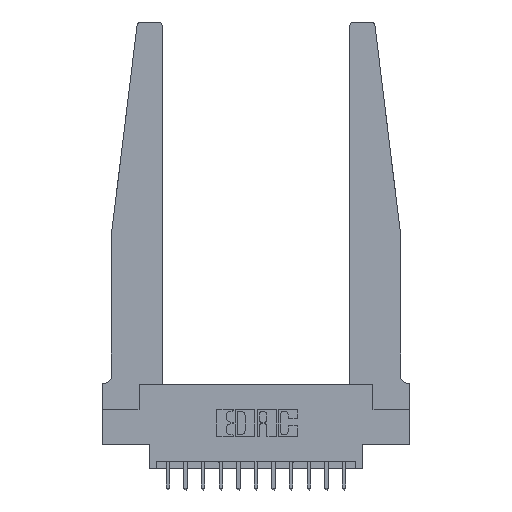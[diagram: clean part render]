
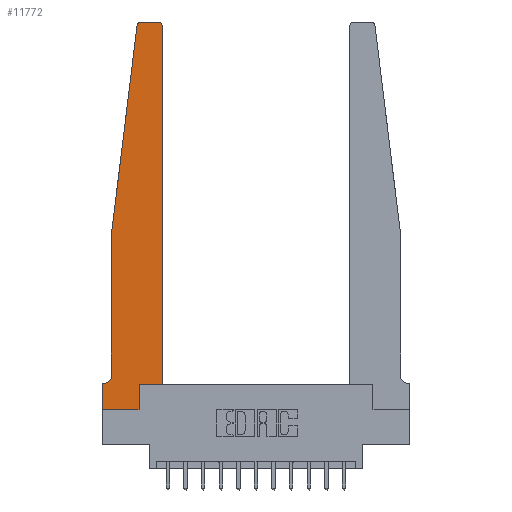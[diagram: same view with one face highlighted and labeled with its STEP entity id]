
A CAD part, top view. The second image highlights one B-rep face of the part: STEP entity #11772.
In plain terms, the highlighted planar face has unit normal (0, 0, 1).
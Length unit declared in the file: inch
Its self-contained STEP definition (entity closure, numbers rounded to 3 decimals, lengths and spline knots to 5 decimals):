
#385 = CARTESIAN_POINT ( 'NONE',  ( 0., 0., 0.37 ) ) ;
#514 = VERTEX_POINT ( 'NONE', #5692 ) ;
#535 = VERTEX_POINT ( 'NONE', #10889 ) ;
#647 = DIRECTION ( 'NONE',  ( 0., 0., -1. ) ) ;
#896 = DIRECTION ( 'NONE',  ( 0., 1., 0. ) ) ;
#1095 = LINE ( 'NONE', #7437, #6168 ) ;
#1302 = EDGE_CURVE ( 'NONE', #15750, #10964, #5642, .T. ) ;
#1675 = VECTOR ( 'NONE', #5531, 39.37008 ) ;
#1702 = VERTEX_POINT ( 'NONE', #1838 ) ;
#1838 = CARTESIAN_POINT ( 'NONE',  ( 0.2605, 0., 0.37 ) ) ;
#1905 = AXIS2_PLACEMENT_3D ( 'NONE', #12193, #647, #10921 ) ;
#1984 = CARTESIAN_POINT ( 'NONE',  ( 0.25, 2.75, 0.37 ) ) ;
#2105 = CARTESIAN_POINT ( 'NONE',  ( 0.2605, 0.18, 0.37 ) ) ;
#2109 = EDGE_CURVE ( 'NONE', #9796, #15750, #9863, .T. ) ;
#2188 = LINE ( 'NONE', #2105, #16376 ) ;
#2191 = VERTEX_POINT ( 'NONE', #4500 ) ;
#2265 = CARTESIAN_POINT ( 'NONE',  ( 0.065, 1.25, 0.37 ) ) ;
#2681 = VERTEX_POINT ( 'NONE', #16068 ) ;
#2759 = CARTESIAN_POINT ( 'NONE',  ( 0., 0., 0.37 ) ) ;
#2778 = VERTEX_POINT ( 'NONE', #15477 ) ;
#2953 = ORIENTED_EDGE ( 'NONE', *, *, #4439, .T. ) ;
#2957 = DIRECTION ( 'NONE',  ( 1., 0., 0. ) ) ;
#3005 = DIRECTION ( 'NONE',  ( -1., 0., 0. ) ) ;
#3137 = AXIS2_PLACEMENT_3D ( 'NONE', #9497, #13600, #11223 ) ;
#3328 = CARTESIAN_POINT ( 'NONE',  ( 0., 0., 0.37 ) ) ;
#3428 = ORIENTED_EDGE ( 'NONE', *, *, #8818, .T. ) ;
#3471 = ORIENTED_EDGE ( 'NONE', *, *, #4637, .T. ) ;
#4064 = EDGE_CURVE ( 'NONE', #535, #14645, #5435, .T. ) ;
#4354 = DIRECTION ( 'NONE',  ( -0.122, -0.992, 0. ) ) ;
#4439 = EDGE_CURVE ( 'NONE', #2778, #2681, #5940, .T. ) ;
#4500 = CARTESIAN_POINT ( 'NONE',  ( 0.2605, 0.18, 0.37 ) ) ;
#4637 = EDGE_CURVE ( 'NONE', #13039, #1702, #6805, .T. ) ;
#5165 = VECTOR ( 'NONE', #10981, 39.37008 ) ;
#5435 = CIRCLE ( 'NONE', #11888, 0.03 ) ;
#5531 = DIRECTION ( 'NONE',  ( 0., -1., 0. ) ) ;
#5535 = ORIENTED_EDGE ( 'NONE', *, *, #8652, .T. ) ;
#5642 = LINE ( 'NONE', #8272, #13247 ) ;
#5692 = CARTESIAN_POINT ( 'NONE',  ( 0.425, 0.18, 0.37 ) ) ;
#5865 = EDGE_CURVE ( 'NONE', #14645, #9796, #16175, .T. ) ;
#5940 = CIRCLE ( 'NONE', #1905, 0.05 ) ;
#6006 = VECTOR ( 'NONE', #13060, 39.37008 ) ;
#6052 = CARTESIAN_POINT ( 'NONE',  ( 0.24675, 2.72367, 0.37 ) ) ;
#6168 = VECTOR ( 'NONE', #16646, 39.37008 ) ;
#6522 = EDGE_CURVE ( 'NONE', #514, #535, #15718, .T. ) ;
#6621 = LINE ( 'NONE', #12861, #8922 ) ;
#6805 = LINE ( 'NONE', #2759, #9969 ) ;
#7226 = LINE ( 'NONE', #385, #1675 ) ;
#7437 = CARTESIAN_POINT ( 'NONE',  ( 0.425, 0.18, 0.37 ) ) ;
#7659 = CARTESIAN_POINT ( 'NONE',  ( 0.395, 2.75, 0.37 ) ) ;
#8180 = ORIENTED_EDGE ( 'NONE', *, *, #5865, .T. ) ;
#8272 = CARTESIAN_POINT ( 'NONE',  ( 0.065, 1.25, 0.37 ) ) ;
#8652 = EDGE_CURVE ( 'NONE', #10964, #2778, #6621, .T. ) ;
#8818 = EDGE_CURVE ( 'NONE', #9942, #13039, #7226, .T. ) ;
#8922 = VECTOR ( 'NONE', #11744, 39.37008 ) ;
#8942 = DIRECTION ( 'NONE',  ( 0., 0., 1. ) ) ;
#9103 = CARTESIAN_POINT ( 'NONE',  ( 0.395, 2.72, 0.37 ) ) ;
#9215 = ORIENTED_EDGE ( 'NONE', *, *, #1302, .T. ) ;
#9420 = LINE ( 'NONE', #14557, #12294 ) ;
#9497 = CARTESIAN_POINT ( 'NONE',  ( 0.27653, 2.72, 0.37 ) ) ;
#9796 = VERTEX_POINT ( 'NONE', #10140 ) ;
#9863 = CIRCLE ( 'NONE', #3137, 0.03 ) ;
#9942 = VERTEX_POINT ( 'NONE', #10730 ) ;
#9969 = VECTOR ( 'NONE', #14473, 39.37008 ) ;
#10069 = EDGE_LOOP ( 'NONE', ( #8180, #12235, #9215, #5535, #2953, #11363, #3428, #3471, #11829, #13147, #10459, #15110 ) ) ;
#10140 = CARTESIAN_POINT ( 'NONE',  ( 0.27653, 2.75, 0.37 ) ) ;
#10459 = ORIENTED_EDGE ( 'NONE', *, *, #6522, .T. ) ;
#10730 = CARTESIAN_POINT ( 'NONE',  ( 0., 0.1875, 0.37 ) ) ;
#10774 = EDGE_CURVE ( 'NONE', #1702, #2191, #2188, .T. ) ;
#10889 = CARTESIAN_POINT ( 'NONE',  ( 0.425, 2.72, 0.37 ) ) ;
#10921 = DIRECTION ( 'NONE',  ( -1., 0., 0. ) ) ;
#10964 = VERTEX_POINT ( 'NONE', #2265 ) ;
#10981 = DIRECTION ( 'NONE',  ( -1., 0., 0. ) ) ;
#11223 = DIRECTION ( 'NONE',  ( 1., 0., 0. ) ) ;
#11363 = ORIENTED_EDGE ( 'NONE', *, *, #13009, .T. ) ;
#11744 = DIRECTION ( 'NONE',  ( 0., -1., 0. ) ) ;
#11772 = ADVANCED_FACE ( 'NONE', ( #14340 ), #15967, .T. ) ;
#11829 = ORIENTED_EDGE ( 'NONE', *, *, #10774, .T. ) ;
#11873 = CARTESIAN_POINT ( 'NONE',  ( 0.425, 0.18, 0.37 ) ) ;
#11888 = AXIS2_PLACEMENT_3D ( 'NONE', #9103, #8942, #16634 ) ;
#12193 = CARTESIAN_POINT ( 'NONE',  ( 0.015, 0.2375, 0.37 ) ) ;
#12235 = ORIENTED_EDGE ( 'NONE', *, *, #2109, .T. ) ;
#12294 = VECTOR ( 'NONE', #3005, 39.37008 ) ;
#12861 = CARTESIAN_POINT ( 'NONE',  ( 0.065, 1.25, 0.37 ) ) ;
#13009 = EDGE_CURVE ( 'NONE', #2681, #9942, #9420, .T. ) ;
#13039 = VERTEX_POINT ( 'NONE', #3328 ) ;
#13060 = DIRECTION ( 'NONE',  ( 0., 1., 0. ) ) ;
#13062 = CARTESIAN_POINT ( 'NONE',  ( 0., 0.1875, 0.37 ) ) ;
#13147 = ORIENTED_EDGE ( 'NONE', *, *, #15438, .T. ) ;
#13247 = VECTOR ( 'NONE', #4354, 39.37008 ) ;
#13600 = DIRECTION ( 'NONE',  ( 0., 0., 1. ) ) ;
#14340 = FACE_OUTER_BOUND ( 'NONE', #10069, .T. ) ;
#14473 = DIRECTION ( 'NONE',  ( 1., 0., 0. ) ) ;
#14557 = CARTESIAN_POINT ( 'NONE',  ( 0.065, 0.1875, 0.37 ) ) ;
#14645 = VERTEX_POINT ( 'NONE', #7659 ) ;
#14674 = DIRECTION ( 'NONE',  ( 0., 0., 1. ) ) ;
#15110 = ORIENTED_EDGE ( 'NONE', *, *, #4064, .T. ) ;
#15438 = EDGE_CURVE ( 'NONE', #2191, #514, #1095, .T. ) ;
#15477 = CARTESIAN_POINT ( 'NONE',  ( 0.065, 0.2375, 0.37 ) ) ;
#15718 = LINE ( 'NONE', #11873, #6006 ) ;
#15750 = VERTEX_POINT ( 'NONE', #6052 ) ;
#15967 = PLANE ( 'NONE',  #16359 ) ;
#16068 = CARTESIAN_POINT ( 'NONE',  ( 0.015, 0.1875, 0.37 ) ) ;
#16175 = LINE ( 'NONE', #1984, #5165 ) ;
#16359 = AXIS2_PLACEMENT_3D ( 'NONE', #13062, #14674, #2957 ) ;
#16376 = VECTOR ( 'NONE', #896, 39.37008 ) ;
#16634 = DIRECTION ( 'NONE',  ( 1., 0., 0. ) ) ;
#16646 = DIRECTION ( 'NONE',  ( 1., 0., 0. ) ) ;
